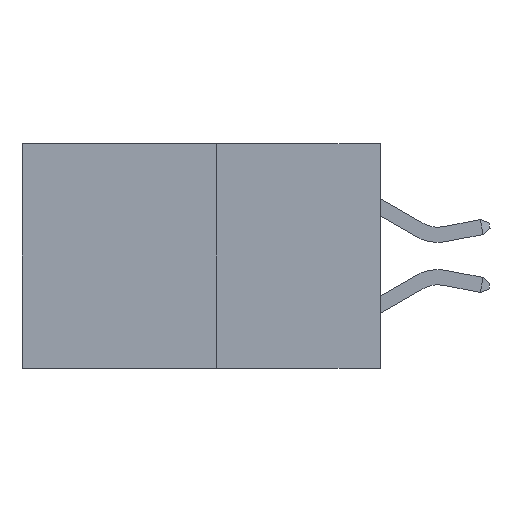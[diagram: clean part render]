
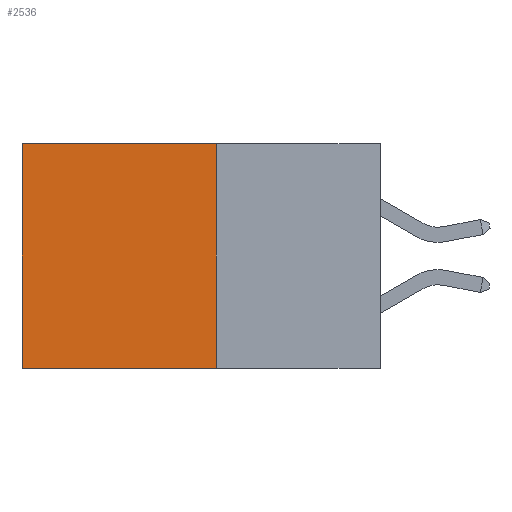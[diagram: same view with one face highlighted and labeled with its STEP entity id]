
A CAD part, left-side view. The second image highlights one B-rep face of the part: STEP entity #2536.
In plain terms, the highlighted planar face has unit normal (-1, 0, 0).
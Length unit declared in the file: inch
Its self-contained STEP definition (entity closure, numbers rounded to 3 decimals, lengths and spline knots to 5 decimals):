
#325 = DIRECTION ( 'NONE',  ( 0., 1., 0. ) ) ;
#347 = VECTOR ( 'NONE', #3533, 39.37008 ) ;
#896 = ORIENTED_EDGE ( 'NONE', *, *, #2944, .T. ) ;
#990 = DIRECTION ( 'NONE',  ( 0., 1., 0. ) ) ;
#1683 = EDGE_CURVE ( 'NONE', #7144, #6519, #2554, .T. ) ;
#1993 = AXIS2_PLACEMENT_3D ( 'NONE', #3583, #3464, #2153 ) ;
#2153 = DIRECTION ( 'NONE',  ( 0., 0., -1. ) ) ;
#2313 = VECTOR ( 'NONE', #990, 39.37008 ) ;
#2536 = ADVANCED_FACE ( 'NONE', ( #6910 ), #3205, .F. ) ;
#2554 = LINE ( 'NONE', #7385, #2313 ) ;
#2601 = EDGE_LOOP ( 'NONE', ( #896, #6616, #8387, #6812 ) ) ;
#2907 = VECTOR ( 'NONE', #8547, 39.37008 ) ;
#2944 = EDGE_CURVE ( 'NONE', #3070, #6519, #3116, .T. ) ;
#3070 = VERTEX_POINT ( 'NONE', #3910 ) ;
#3116 = LINE ( 'NONE', #7575, #2907 ) ;
#3205 = PLANE ( 'NONE',  #1993 ) ;
#3464 = DIRECTION ( 'NONE',  ( 1., 0., 0. ) ) ;
#3533 = DIRECTION ( 'NONE',  ( 0., 0., -1. ) ) ;
#3583 = CARTESIAN_POINT ( 'NONE',  ( 0.277, 0.27, -0.37 ) ) ;
#3910 = CARTESIAN_POINT ( 'NONE',  ( 0.277, 0.59, 0. ) ) ;
#3956 = CARTESIAN_POINT ( 'NONE',  ( 0.277, 0.27, 0. ) ) ;
#4190 = LINE ( 'NONE', #8972, #347 ) ;
#4727 = VECTOR ( 'NONE', #325, 39.37008 ) ;
#4786 = VERTEX_POINT ( 'NONE', #8197 ) ;
#5133 = CARTESIAN_POINT ( 'NONE',  ( 0.277, 0.27, -0.37 ) ) ;
#6519 = VERTEX_POINT ( 'NONE', #7840 ) ;
#6616 = ORIENTED_EDGE ( 'NONE', *, *, #1683, .F. ) ;
#6812 = ORIENTED_EDGE ( 'NONE', *, *, #8274, .T. ) ;
#6910 = FACE_OUTER_BOUND ( 'NONE', #2601, .T. ) ;
#7144 = VERTEX_POINT ( 'NONE', #5133 ) ;
#7385 = CARTESIAN_POINT ( 'NONE',  ( 0.277, 0.27, -0.37 ) ) ;
#7575 = CARTESIAN_POINT ( 'NONE',  ( 0.277, 0.59, -0.37 ) ) ;
#7840 = CARTESIAN_POINT ( 'NONE',  ( 0.277, 0.59, -0.37 ) ) ;
#8197 = CARTESIAN_POINT ( 'NONE',  ( 0.277, 0.27, 0. ) ) ;
#8274 = EDGE_CURVE ( 'NONE', #4786, #3070, #8627, .T. ) ;
#8387 = ORIENTED_EDGE ( 'NONE', *, *, #8608, .F. ) ;
#8547 = DIRECTION ( 'NONE',  ( 0., 0., -1. ) ) ;
#8608 = EDGE_CURVE ( 'NONE', #4786, #7144, #4190, .T. ) ;
#8627 = LINE ( 'NONE', #3956, #4727 ) ;
#8972 = CARTESIAN_POINT ( 'NONE',  ( 0.277, 0.27, -0.37 ) ) ;
